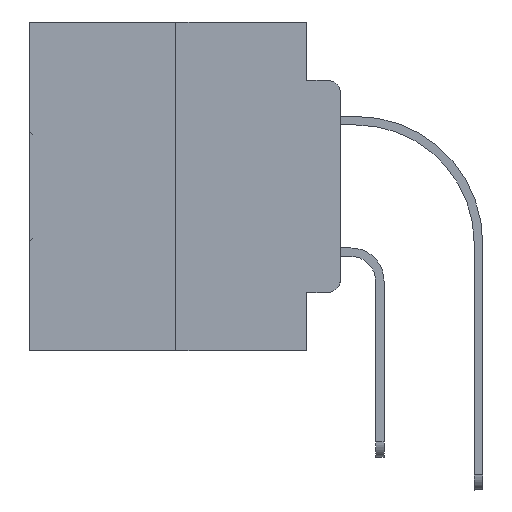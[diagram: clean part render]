
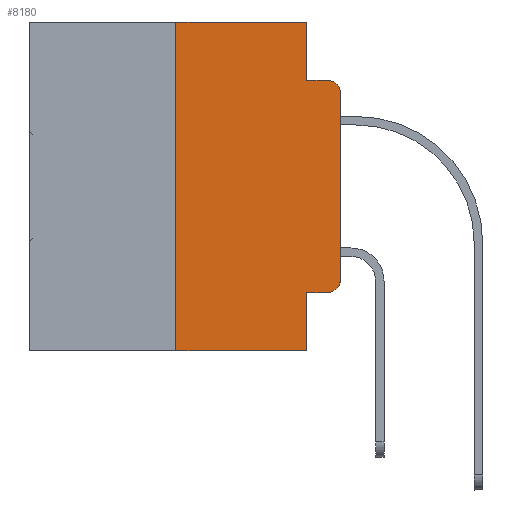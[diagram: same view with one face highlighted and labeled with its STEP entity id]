
A CAD part, left-side view. The second image highlights one B-rep face of the part: STEP entity #8180.
In plain terms, the highlighted planar face has unit normal (-1, 0, 0).
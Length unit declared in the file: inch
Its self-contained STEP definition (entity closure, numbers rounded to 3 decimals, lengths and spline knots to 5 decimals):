
#19 = DIRECTION ( 'NONE',  ( 0., -1., 0. ) ) ;
#150 = CARTESIAN_POINT ( 'NONE',  ( 0., 0.02, -0.3915 ) ) ;
#327 = LINE ( 'NONE', #25880, #672 ) ;
#672 = VECTOR ( 'NONE', #7343, 39.37008 ) ;
#739 = LINE ( 'NONE', #19490, #16450 ) ;
#1361 = VERTEX_POINT ( 'NONE', #26828 ) ;
#1814 = VERTEX_POINT ( 'NONE', #29717 ) ;
#3188 = VECTOR ( 'NONE', #18127, 39.37008 ) ;
#3218 = ORIENTED_EDGE ( 'NONE', *, *, #27694, .T. ) ;
#3395 = ORIENTED_EDGE ( 'NONE', *, *, #17116, .F. ) ;
#3629 = CARTESIAN_POINT ( 'NONE',  ( 0., 0., -0.3915 ) ) ;
#3908 = AXIS2_PLACEMENT_3D ( 'NONE', #21332, #26336, #26182 ) ;
#4004 = VERTEX_POINT ( 'NONE', #29543 ) ;
#4060 = ORIENTED_EDGE ( 'NONE', *, *, #26867, .T. ) ;
#4095 = DIRECTION ( 'NONE',  ( 0., 0., -1. ) ) ;
#4352 = EDGE_CURVE ( 'NONE', #11485, #4677, #327, .T. ) ;
#4442 = LINE ( 'NONE', #33209, #27609 ) ;
#4677 = VERTEX_POINT ( 'NONE', #7775 ) ;
#5571 = CIRCLE ( 'NONE', #3908, 0.02 ) ;
#5872 = CARTESIAN_POINT ( 'NONE',  ( 0., 0.473, 0. ) ) ;
#6137 = CIRCLE ( 'NONE', #33238, 0.02 ) ;
#6326 = VERTEX_POINT ( 'NONE', #9489 ) ;
#6572 = VERTEX_POINT ( 'NONE', #8431 ) ;
#6604 = LINE ( 'NONE', #33273, #23231 ) ;
#7343 = DIRECTION ( 'NONE',  ( 0., 0., 1. ) ) ;
#7775 = CARTESIAN_POINT ( 'NONE',  ( 0., 0.25, 0. ) ) ;
#8180 = ADVANCED_FACE ( 'NONE', ( #11426 ), #19430, .F. ) ;
#8225 = VERTEX_POINT ( 'NONE', #30990 ) ;
#8431 = CARTESIAN_POINT ( 'NONE',  ( 0., 0.02, -0.4115 ) ) ;
#9159 = CARTESIAN_POINT ( 'NONE',  ( 0., 0.051, 0. ) ) ;
#9489 = CARTESIAN_POINT ( 'NONE',  ( 0., 0.051, -0.5 ) ) ;
#9714 = VERTEX_POINT ( 'NONE', #31506 ) ;
#10903 = DIRECTION ( 'NONE',  ( -1., 0., 0. ) ) ;
#11207 = EDGE_LOOP ( 'NONE', ( #31845, #17795, #14307, #13055, #3395, #32626, #4060, #20424, #3218, #19394 ) ) ;
#11426 = FACE_OUTER_BOUND ( 'NONE', #11207, .T. ) ;
#11485 = VERTEX_POINT ( 'NONE', #27979 ) ;
#11591 = LINE ( 'NONE', #9159, #20652 ) ;
#13055 = ORIENTED_EDGE ( 'NONE', *, *, #24169, .F. ) ;
#14307 = ORIENTED_EDGE ( 'NONE', *, *, #26016, .F. ) ;
#14404 = LINE ( 'NONE', #27400, #32597 ) ;
#15295 = CARTESIAN_POINT ( 'NONE',  ( 0., 0.051, -0.0885 ) ) ;
#16450 = VECTOR ( 'NONE', #29360, 39.37008 ) ;
#17116 = EDGE_CURVE ( 'NONE', #4677, #1814, #14404, .T. ) ;
#17371 = DIRECTION ( 'NONE',  ( 0., -1., 0. ) ) ;
#17795 = ORIENTED_EDGE ( 'NONE', *, *, #22491, .T. ) ;
#18127 = DIRECTION ( 'NONE',  ( 0., -1., 0. ) ) ;
#18134 = VECTOR ( 'NONE', #19, 39.37008 ) ;
#18874 = AXIS2_PLACEMENT_3D ( 'NONE', #5872, #19252, #19600 ) ;
#19252 = DIRECTION ( 'NONE',  ( 1., 0., 0. ) ) ;
#19394 = ORIENTED_EDGE ( 'NONE', *, *, #22618, .T. ) ;
#19430 = PLANE ( 'NONE',  #18874 ) ;
#19490 = CARTESIAN_POINT ( 'NONE',  ( 0., 0., 0. ) ) ;
#19600 = DIRECTION ( 'NONE',  ( 0., 0., -1. ) ) ;
#20424 = ORIENTED_EDGE ( 'NONE', *, *, #24999, .F. ) ;
#20514 = LINE ( 'NONE', #15295, #18134 ) ;
#20652 = VECTOR ( 'NONE', #30295, 39.37008 ) ;
#21332 = CARTESIAN_POINT ( 'NONE',  ( 0., 0.02, -0.1085 ) ) ;
#21512 = DIRECTION ( 'NONE',  ( 0., 0., -1. ) ) ;
#22491 = EDGE_CURVE ( 'NONE', #4004, #1361, #5571, .T. ) ;
#22618 = EDGE_CURVE ( 'NONE', #6572, #28977, #6137, .T. ) ;
#23231 = VECTOR ( 'NONE', #17371, 39.37008 ) ;
#23524 = CARTESIAN_POINT ( 'NONE',  ( 0., 0.473, -0.5 ) ) ;
#24169 = EDGE_CURVE ( 'NONE', #1814, #9714, #11591, .T. ) ;
#24999 = EDGE_CURVE ( 'NONE', #8225, #6326, #4442, .T. ) ;
#25691 = EDGE_CURVE ( 'NONE', #28977, #4004, #739, .T. ) ;
#25880 = CARTESIAN_POINT ( 'NONE',  ( 0., 0.25, 0. ) ) ;
#26016 = EDGE_CURVE ( 'NONE', #9714, #1361, #20514, .T. ) ;
#26182 = DIRECTION ( 'NONE',  ( 0., 0., -1. ) ) ;
#26336 = DIRECTION ( 'NONE',  ( -1., 0., 0. ) ) ;
#26828 = CARTESIAN_POINT ( 'NONE',  ( 0., 0.02, -0.0885 ) ) ;
#26867 = EDGE_CURVE ( 'NONE', #11485, #6326, #31622, .T. ) ;
#27400 = CARTESIAN_POINT ( 'NONE',  ( 0., 0.473, 0. ) ) ;
#27609 = VECTOR ( 'NONE', #4095, 39.37008 ) ;
#27694 = EDGE_CURVE ( 'NONE', #8225, #6572, #6604, .T. ) ;
#27979 = CARTESIAN_POINT ( 'NONE',  ( 0., 0.25, -0.5 ) ) ;
#28977 = VERTEX_POINT ( 'NONE', #3629 ) ;
#29358 = DIRECTION ( 'NONE',  ( 0., -1., 0. ) ) ;
#29360 = DIRECTION ( 'NONE',  ( 0., 0., 1. ) ) ;
#29543 = CARTESIAN_POINT ( 'NONE',  ( 0., 0., -0.1085 ) ) ;
#29717 = CARTESIAN_POINT ( 'NONE',  ( 0., 0.051, 0. ) ) ;
#30295 = DIRECTION ( 'NONE',  ( 0., 0., -1. ) ) ;
#30990 = CARTESIAN_POINT ( 'NONE',  ( 0., 0.051, -0.4115 ) ) ;
#31506 = CARTESIAN_POINT ( 'NONE',  ( 0., 0.051, -0.0885 ) ) ;
#31622 = LINE ( 'NONE', #23524, #3188 ) ;
#31845 = ORIENTED_EDGE ( 'NONE', *, *, #25691, .T. ) ;
#32597 = VECTOR ( 'NONE', #29358, 39.37008 ) ;
#32626 = ORIENTED_EDGE ( 'NONE', *, *, #4352, .F. ) ;
#33209 = CARTESIAN_POINT ( 'NONE',  ( 0., 0.051, 0. ) ) ;
#33238 = AXIS2_PLACEMENT_3D ( 'NONE', #150, #10903, #21512 ) ;
#33273 = CARTESIAN_POINT ( 'NONE',  ( 0., 0.051, -0.4115 ) ) ;
